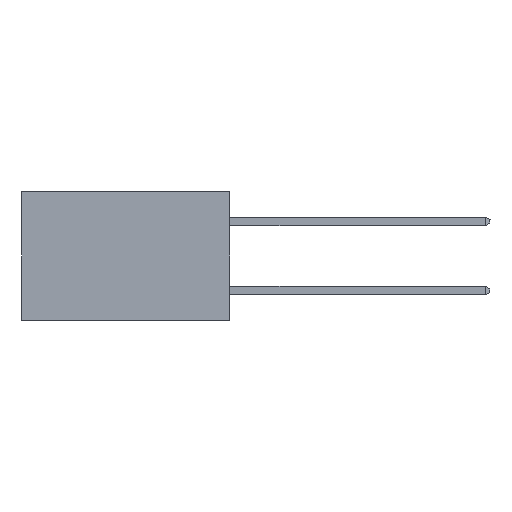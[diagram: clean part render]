
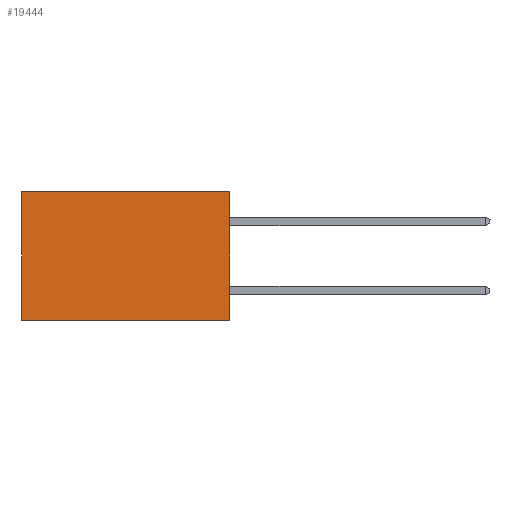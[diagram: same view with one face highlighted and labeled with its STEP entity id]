
A CAD part, left-side view. The second image highlights one B-rep face of the part: STEP entity #19444.
In plain terms, the highlighted planar face has unit normal (-1, 0, 0).
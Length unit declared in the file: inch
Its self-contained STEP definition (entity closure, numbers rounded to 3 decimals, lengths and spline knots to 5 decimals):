
#583 = CARTESIAN_POINT ( 'NONE',  ( 0.298, 0., -0.37 ) ) ;
#1906 = EDGE_LOOP ( 'NONE', ( #30055, #26553, #26528, #18093 ) ) ;
#1930 = DIRECTION ( 'NONE',  ( 0., 1., 0. ) ) ;
#2909 = LINE ( 'NONE', #9915, #8560 ) ;
#4595 = FACE_OUTER_BOUND ( 'NONE', #1906, .T. ) ;
#4891 = VECTOR ( 'NONE', #14022, 39.37008 ) ;
#5125 = DIRECTION ( 'NONE',  ( 0., 0., -1. ) ) ;
#6336 = EDGE_CURVE ( 'NONE', #28359, #22228, #23956, .T. ) ;
#6815 = EDGE_CURVE ( 'NONE', #11478, #28359, #24358, .T. ) ;
#6842 = CARTESIAN_POINT ( 'NONE',  ( 0.298, 0.6, 0. ) ) ;
#8560 = VECTOR ( 'NONE', #5125, 39.37008 ) ;
#8949 = VECTOR ( 'NONE', #1930, 39.37008 ) ;
#9908 = CARTESIAN_POINT ( 'NONE',  ( 0.298, 0., 0. ) ) ;
#9915 = CARTESIAN_POINT ( 'NONE',  ( 0.298, 0., 0. ) ) ;
#11478 = VERTEX_POINT ( 'NONE', #17561 ) ;
#11542 = VECTOR ( 'NONE', #18256, 39.37008 ) ;
#11731 = EDGE_CURVE ( 'NONE', #19476, #22228, #28905, .T. ) ;
#12238 = DIRECTION ( 'NONE',  ( 1., 0., 0. ) ) ;
#14022 = DIRECTION ( 'NONE',  ( 0., 1., 0. ) ) ;
#15521 = AXIS2_PLACEMENT_3D ( 'NONE', #9908, #12238, #28509 ) ;
#16112 = CARTESIAN_POINT ( 'NONE',  ( 0.298, 0., -0.37 ) ) ;
#17561 = CARTESIAN_POINT ( 'NONE',  ( 0.298, 0., 0. ) ) ;
#18093 = ORIENTED_EDGE ( 'NONE', *, *, #6815, .T. ) ;
#18256 = DIRECTION ( 'NONE',  ( 0., 0., -1. ) ) ;
#19444 = ADVANCED_FACE ( 'NONE', ( #4595 ), #23883, .F. ) ;
#19476 = VERTEX_POINT ( 'NONE', #583 ) ;
#21280 = CARTESIAN_POINT ( 'NONE',  ( 0.298, 0., 0. ) ) ;
#21364 = EDGE_CURVE ( 'NONE', #11478, #19476, #2909, .T. ) ;
#22228 = VERTEX_POINT ( 'NONE', #24459 ) ;
#23883 = PLANE ( 'NONE',  #15521 ) ;
#23956 = LINE ( 'NONE', #29311, #11542 ) ;
#24358 = LINE ( 'NONE', #21280, #4891 ) ;
#24459 = CARTESIAN_POINT ( 'NONE',  ( 0.298, 0.6, -0.37 ) ) ;
#26528 = ORIENTED_EDGE ( 'NONE', *, *, #21364, .F. ) ;
#26553 = ORIENTED_EDGE ( 'NONE', *, *, #11731, .F. ) ;
#28359 = VERTEX_POINT ( 'NONE', #6842 ) ;
#28509 = DIRECTION ( 'NONE',  ( 0., 0., -1. ) ) ;
#28905 = LINE ( 'NONE', #16112, #8949 ) ;
#29311 = CARTESIAN_POINT ( 'NONE',  ( 0.298, 0.6, 0. ) ) ;
#30055 = ORIENTED_EDGE ( 'NONE', *, *, #6336, .T. ) ;
